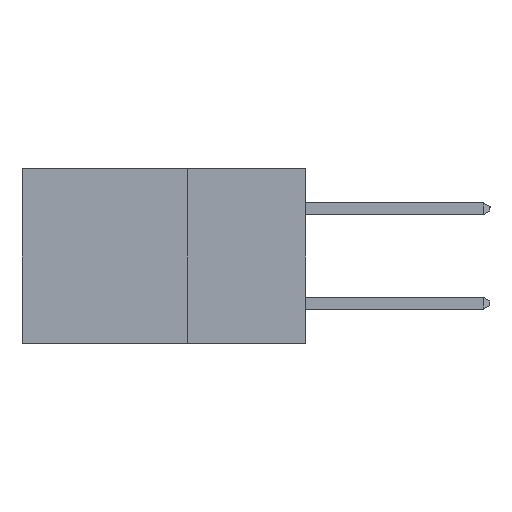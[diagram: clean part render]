
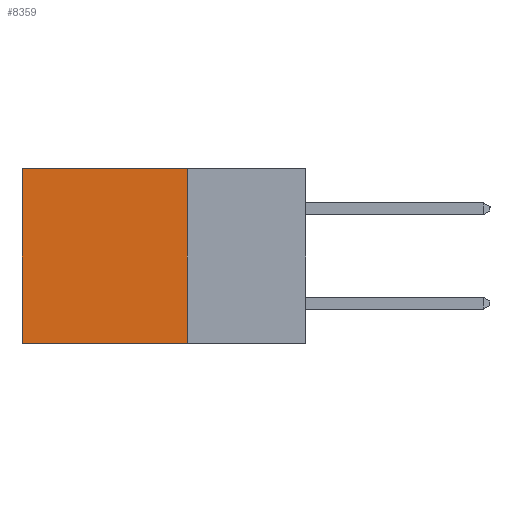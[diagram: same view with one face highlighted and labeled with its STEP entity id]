
A CAD part, left-side view. The second image highlights one B-rep face of the part: STEP entity #8359.
In plain terms, the highlighted planar face has unit normal (-1, 0, 0).
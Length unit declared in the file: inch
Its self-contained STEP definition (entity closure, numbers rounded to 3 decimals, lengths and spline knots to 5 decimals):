
#372 = DIRECTION ( 'NONE',  ( 0., 1., 0. ) ) ;
#456 = DIRECTION ( 'NONE',  ( 0., 0., -1. ) ) ;
#1044 = ORIENTED_EDGE ( 'NONE', *, *, #5950, .F. ) ;
#1125 = DIRECTION ( 'NONE',  ( 0., 1., 0. ) ) ;
#1155 = LINE ( 'NONE', #1305, #6321 ) ;
#1288 = LINE ( 'NONE', #5516, #2652 ) ;
#1305 = CARTESIAN_POINT ( 'NONE',  ( 0.2615, 0.25, 0. ) ) ;
#1959 = DIRECTION ( 'NONE',  ( 0., 0., -1. ) ) ;
#2340 = VERTEX_POINT ( 'NONE', #8256 ) ;
#2535 = DIRECTION ( 'NONE',  ( 0., 0., -1. ) ) ;
#2652 = VECTOR ( 'NONE', #456, 39.37008 ) ;
#2950 = CARTESIAN_POINT ( 'NONE',  ( 0.2615, 0.25, 0. ) ) ;
#2992 = VERTEX_POINT ( 'NONE', #7947 ) ;
#3016 = EDGE_LOOP ( 'NONE', ( #7785, #1044, #4463, #4369 ) ) ;
#3291 = FACE_OUTER_BOUND ( 'NONE', #3016, .T. ) ;
#3350 = EDGE_CURVE ( 'NONE', #5174, #5064, #1155, .T. ) ;
#4004 = LINE ( 'NONE', #5052, #9568 ) ;
#4080 = CARTESIAN_POINT ( 'NONE',  ( 0.2615, 0.25, -0.37 ) ) ;
#4369 = ORIENTED_EDGE ( 'NONE', *, *, #3350, .T. ) ;
#4463 = ORIENTED_EDGE ( 'NONE', *, *, #8409, .F. ) ;
#5052 = CARTESIAN_POINT ( 'NONE',  ( 0.2615, 0.25, -0.37 ) ) ;
#5064 = VERTEX_POINT ( 'NONE', #9429 ) ;
#5174 = VERTEX_POINT ( 'NONE', #2950 ) ;
#5273 = VECTOR ( 'NONE', #2535, 39.37008 ) ;
#5516 = CARTESIAN_POINT ( 'NONE',  ( 0.2615, 0.25, -0.37 ) ) ;
#5950 = EDGE_CURVE ( 'NONE', #2992, #2340, #4004, .T. ) ;
#6225 = LINE ( 'NONE', #7724, #5273 ) ;
#6321 = VECTOR ( 'NONE', #372, 39.37008 ) ;
#6523 = AXIS2_PLACEMENT_3D ( 'NONE', #4080, #8599, #1959 ) ;
#7519 = EDGE_CURVE ( 'NONE', #5064, #2340, #6225, .T. ) ;
#7724 = CARTESIAN_POINT ( 'NONE',  ( 0.2615, 0.6, -0.37 ) ) ;
#7785 = ORIENTED_EDGE ( 'NONE', *, *, #7519, .T. ) ;
#7883 = PLANE ( 'NONE',  #6523 ) ;
#7947 = CARTESIAN_POINT ( 'NONE',  ( 0.2615, 0.25, -0.37 ) ) ;
#8256 = CARTESIAN_POINT ( 'NONE',  ( 0.2615, 0.6, -0.37 ) ) ;
#8359 = ADVANCED_FACE ( 'NONE', ( #3291 ), #7883, .F. ) ;
#8409 = EDGE_CURVE ( 'NONE', #5174, #2992, #1288, .T. ) ;
#8599 = DIRECTION ( 'NONE',  ( 1., 0., 0. ) ) ;
#9429 = CARTESIAN_POINT ( 'NONE',  ( 0.2615, 0.6, 0. ) ) ;
#9568 = VECTOR ( 'NONE', #1125, 39.37008 ) ;
